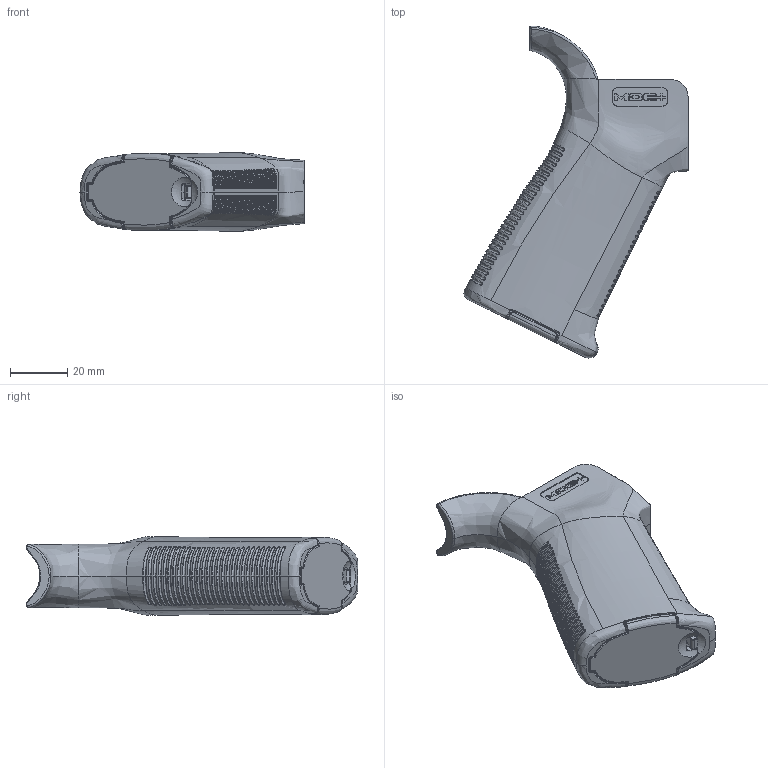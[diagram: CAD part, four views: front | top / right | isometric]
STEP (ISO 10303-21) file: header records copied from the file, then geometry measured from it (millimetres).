
FILE_DESCRIPTION( ( '' ), ' ' );
FILE_NAME( '5a11559d45e0160f24f889ed.step', '2017-11-19T09:58:03', ( '' ), ( '' ), ' ', ' ', ' ' );
FILE_SCHEMA( ( 'AUTOMOTIVE_DESIGN { 1 0 10303 214 1 1 1 1 }' ) );
Length unit declared in the file: metre
Products named in the file (1): Part 1
Bounding box: 78.08 x 115.71 x 27.45 mm (x, y, z)
Volume: 53104.1 mm3; surface area: 24626.3 mm2
Topology: 1 solids, 1 shells, 580 faces, 1476 edges, 949 vertices
Faces by surface type: bspline 337, plane 160, cylinder 57, extrusion 16, torus 8, revolution 2
Full cylindrical faces by diameter (mm): 2.997 x1, 7.112 x1, 7.62 x1
Entity records: 170443 total; most frequent: CARTESIAN_POINT 154908, ORIENTED_EDGE 2936, EDGE_CURVE 1468, DIRECTION 1149, B_SPLINE_CURVE_WITH_KNOTS 995, VERTEX_POINT 948, EDGE_LOOP 652, FACE_OUTER_BOUND 583
